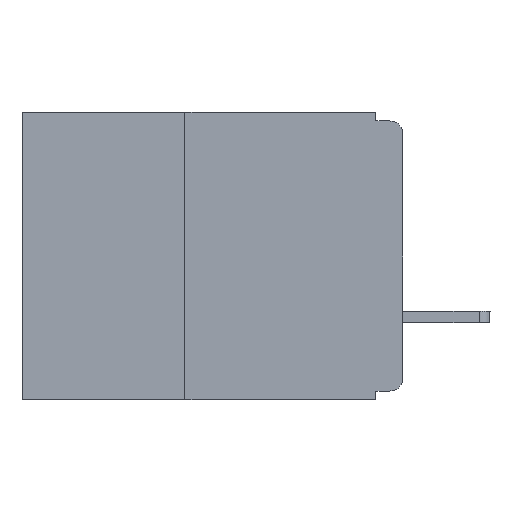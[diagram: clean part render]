
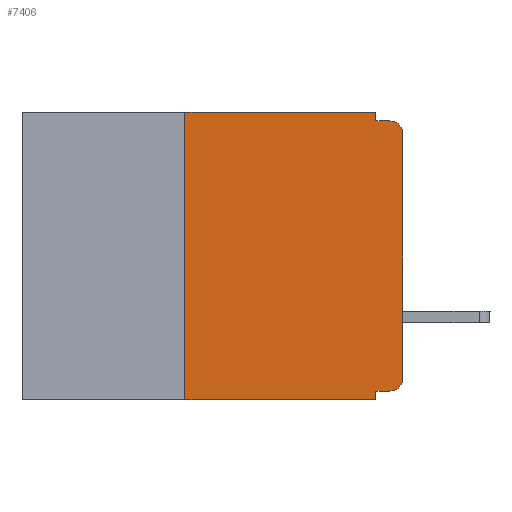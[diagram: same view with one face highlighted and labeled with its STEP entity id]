
A CAD part, left-side view. The second image highlights one B-rep face of the part: STEP entity #7406.
In plain terms, the highlighted planar face has unit normal (-1, 0, 0).
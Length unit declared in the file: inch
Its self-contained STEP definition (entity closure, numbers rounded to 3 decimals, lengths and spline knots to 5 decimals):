
#80 = CARTESIAN_POINT ( 'NONE',  ( 0., 0.437, 0. ) ) ;
#104 = VERTEX_POINT ( 'NONE', #4214 ) ;
#150 = ORIENTED_EDGE ( 'NONE', *, *, #4117, .F. ) ;
#297 = DIRECTION ( 'NONE',  ( -1., 0., 0. ) ) ;
#504 = CIRCLE ( 'NONE', #2575, 0.015 ) ;
#811 = VERTEX_POINT ( 'NONE', #10148 ) ;
#877 = CARTESIAN_POINT ( 'NONE',  ( 0., 0.015, -0.01 ) ) ;
#1176 = CARTESIAN_POINT ( 'NONE',  ( 0., 0.437, -0.33 ) ) ;
#1179 = DIRECTION ( 'NONE',  ( 0., 1., 0. ) ) ;
#1276 = LINE ( 'NONE', #9141, #13375 ) ;
#1289 = VERTEX_POINT ( 'NONE', #6824 ) ;
#1294 = CARTESIAN_POINT ( 'NONE',  ( 0., 0.25, 0. ) ) ;
#1681 = ORIENTED_EDGE ( 'NONE', *, *, #7178, .F. ) ;
#2087 = CARTESIAN_POINT ( 'NONE',  ( 0., 0., -0.32 ) ) ;
#2111 = DIRECTION ( 'NONE',  ( 0., -1., 0. ) ) ;
#2526 = EDGE_CURVE ( 'NONE', #1289, #8401, #2736, .T. ) ;
#2575 = AXIS2_PLACEMENT_3D ( 'NONE', #7446, #3230, #8572 ) ;
#2736 = LINE ( 'NONE', #1176, #13454 ) ;
#2834 = EDGE_CURVE ( 'NONE', #8464, #6837, #504, .T. ) ;
#3019 = ORIENTED_EDGE ( 'NONE', *, *, #7603, .F. ) ;
#3230 = DIRECTION ( 'NONE',  ( -1., 0., 0. ) ) ;
#3300 = DIRECTION ( 'NONE',  ( 0., -1., 0. ) ) ;
#3598 = ORIENTED_EDGE ( 'NONE', *, *, #12342, .T. ) ;
#3608 = ORIENTED_EDGE ( 'NONE', *, *, #12793, .F. ) ;
#3847 = DIRECTION ( 'NONE',  ( 0., 0., -1. ) ) ;
#4046 = CARTESIAN_POINT ( 'NONE',  ( 0., 0., -0.01 ) ) ;
#4117 = EDGE_CURVE ( 'NONE', #10160, #811, #7930, .T. ) ;
#4214 = CARTESIAN_POINT ( 'NONE',  ( 0., 0., -0.025 ) ) ;
#4535 = VECTOR ( 'NONE', #3847, 39.37008 ) ;
#4855 = CARTESIAN_POINT ( 'NONE',  ( 0., 0.031, 0. ) ) ;
#5089 = CARTESIAN_POINT ( 'NONE',  ( 0., 0.437, 0. ) ) ;
#5192 = EDGE_LOOP ( 'NONE', ( #5820, #3598, #1681, #150, #3019, #13391, #9409, #5922, #3608, #10534 ) ) ;
#5635 = EDGE_CURVE ( 'NONE', #1289, #9743, #11330, .T. ) ;
#5730 = CARTESIAN_POINT ( 'NONE',  ( 0., 0.015, -0.025 ) ) ;
#5820 = ORIENTED_EDGE ( 'NONE', *, *, #5867, .T. ) ;
#5867 = EDGE_CURVE ( 'NONE', #6837, #104, #1276, .T. ) ;
#5922 = ORIENTED_EDGE ( 'NONE', *, *, #6938, .F. ) ;
#6501 = VERTEX_POINT ( 'NONE', #877 ) ;
#6794 = LINE ( 'NONE', #2087, #11936 ) ;
#6824 = CARTESIAN_POINT ( 'NONE',  ( 0., 0.25, -0.33 ) ) ;
#6837 = VERTEX_POINT ( 'NONE', #8450 ) ;
#6869 = DIRECTION ( 'NONE',  ( 0., 0., 1. ) ) ;
#6938 = EDGE_CURVE ( 'NONE', #14045, #8401, #8204, .T. ) ;
#7178 = EDGE_CURVE ( 'NONE', #811, #6501, #10583, .T. ) ;
#7406 = ADVANCED_FACE ( 'NONE', ( #8541 ), #10946, .F. ) ;
#7446 = CARTESIAN_POINT ( 'NONE',  ( 0., 0.015, -0.305 ) ) ;
#7603 = EDGE_CURVE ( 'NONE', #9743, #10160, #11253, .T. ) ;
#7644 = DIRECTION ( 'NONE',  ( 0., 0., -1. ) ) ;
#7930 = LINE ( 'NONE', #4855, #4535 ) ;
#8204 = LINE ( 'NONE', #9119, #13331 ) ;
#8339 = AXIS2_PLACEMENT_3D ( 'NONE', #80, #11037, #7644 ) ;
#8401 = VERTEX_POINT ( 'NONE', #10250 ) ;
#8450 = CARTESIAN_POINT ( 'NONE',  ( 0., 0., -0.305 ) ) ;
#8464 = VERTEX_POINT ( 'NONE', #10391 ) ;
#8541 = FACE_OUTER_BOUND ( 'NONE', #5192, .T. ) ;
#8572 = DIRECTION ( 'NONE',  ( 0., 0., -1. ) ) ;
#8938 = VECTOR ( 'NONE', #9795, 39.37008 ) ;
#9119 = CARTESIAN_POINT ( 'NONE',  ( 0., 0.031, -0.33 ) ) ;
#9141 = CARTESIAN_POINT ( 'NONE',  ( 0., 0., 0. ) ) ;
#9174 = CARTESIAN_POINT ( 'NONE',  ( 0., 0.031, -0.32 ) ) ;
#9409 = ORIENTED_EDGE ( 'NONE', *, *, #2526, .T. ) ;
#9743 = VERTEX_POINT ( 'NONE', #1294 ) ;
#9795 = DIRECTION ( 'NONE',  ( 0., 0., 1. ) ) ;
#9994 = DIRECTION ( 'NONE',  ( 0., 0., -1. ) ) ;
#10148 = CARTESIAN_POINT ( 'NONE',  ( 0., 0.031, -0.01 ) ) ;
#10160 = VERTEX_POINT ( 'NONE', #11666 ) ;
#10250 = CARTESIAN_POINT ( 'NONE',  ( 0., 0.031, -0.33 ) ) ;
#10391 = CARTESIAN_POINT ( 'NONE',  ( 0., 0.015, -0.32 ) ) ;
#10534 = ORIENTED_EDGE ( 'NONE', *, *, #2834, .T. ) ;
#10583 = LINE ( 'NONE', #4046, #11956 ) ;
#10946 = PLANE ( 'NONE',  #8339 ) ;
#11024 = AXIS2_PLACEMENT_3D ( 'NONE', #5730, #297, #13462 ) ;
#11037 = DIRECTION ( 'NONE',  ( 1., 0., 0. ) ) ;
#11253 = LINE ( 'NONE', #5089, #13831 ) ;
#11330 = LINE ( 'NONE', #13872, #8938 ) ;
#11580 = DIRECTION ( 'NONE',  ( 0., -1., 0. ) ) ;
#11666 = CARTESIAN_POINT ( 'NONE',  ( 0., 0.031, 0. ) ) ;
#11936 = VECTOR ( 'NONE', #1179, 39.37008 ) ;
#11956 = VECTOR ( 'NONE', #11580, 39.37008 ) ;
#12342 = EDGE_CURVE ( 'NONE', #104, #6501, #13323, .T. ) ;
#12793 = EDGE_CURVE ( 'NONE', #8464, #14045, #6794, .T. ) ;
#13323 = CIRCLE ( 'NONE', #11024, 0.015 ) ;
#13331 = VECTOR ( 'NONE', #9994, 39.37008 ) ;
#13375 = VECTOR ( 'NONE', #6869, 39.37008 ) ;
#13391 = ORIENTED_EDGE ( 'NONE', *, *, #5635, .F. ) ;
#13454 = VECTOR ( 'NONE', #3300, 39.37008 ) ;
#13462 = DIRECTION ( 'NONE',  ( 0., 0., -1. ) ) ;
#13831 = VECTOR ( 'NONE', #2111, 39.37008 ) ;
#13872 = CARTESIAN_POINT ( 'NONE',  ( 0., 0.25, -0.33 ) ) ;
#14045 = VERTEX_POINT ( 'NONE', #9174 ) ;
